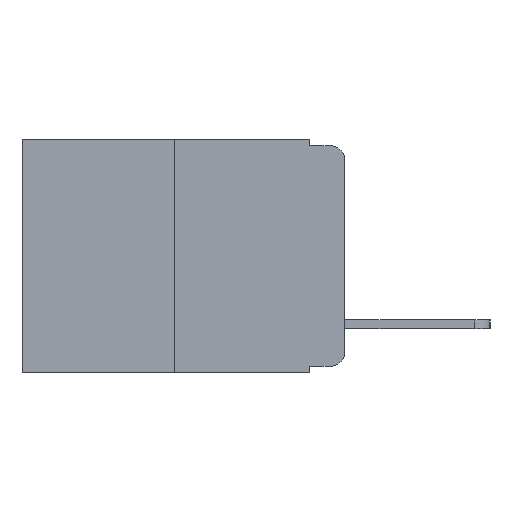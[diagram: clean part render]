
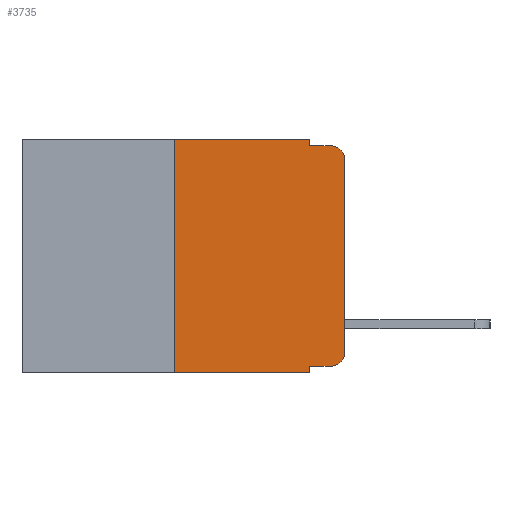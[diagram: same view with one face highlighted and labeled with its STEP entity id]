
A CAD part, left-side view. The second image highlights one B-rep face of the part: STEP entity #3735.
In plain terms, the highlighted planar face has unit normal (-1, 0, 0).
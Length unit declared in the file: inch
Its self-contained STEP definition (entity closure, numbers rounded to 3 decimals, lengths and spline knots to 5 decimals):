
#361 = FACE_OUTER_BOUND ( 'NONE', #10291, .T. ) ;
#640 = LINE ( 'NONE', #11534, #10265 ) ;
#1493 = ORIENTED_EDGE ( 'NONE', *, *, #13781, .T. ) ;
#2721 = EDGE_CURVE ( 'NONE', #24063, #6639, #3100, .T. ) ;
#3065 = ORIENTED_EDGE ( 'NONE', *, *, #8632, .F. ) ;
#3100 = CIRCLE ( 'NONE', #19921, 0.02 ) ;
#3226 = LINE ( 'NONE', #7945, #12706 ) ;
#3735 = ADVANCED_FACE ( 'NONE', ( #361 ), #19083, .F. ) ;
#3847 = DIRECTION ( 'NONE',  ( 0., 0., -1. ) ) ;
#4393 = DIRECTION ( 'NONE',  ( 0., -1., 0. ) ) ;
#4497 = CARTESIAN_POINT ( 'NONE',  ( 0., 0.051, 0. ) ) ;
#4595 = DIRECTION ( 'NONE',  ( 0., -1., 0. ) ) ;
#5886 = CARTESIAN_POINT ( 'NONE',  ( 0., 0.051, -0.333 ) ) ;
#6579 = VECTOR ( 'NONE', #8609, 39.37008 ) ;
#6639 = VERTEX_POINT ( 'NONE', #22176 ) ;
#6747 = CARTESIAN_POINT ( 'NONE',  ( 0., 0.473, 0. ) ) ;
#7032 = ORIENTED_EDGE ( 'NONE', *, *, #11945, .T. ) ;
#7198 = ORIENTED_EDGE ( 'NONE', *, *, #11677, .T. ) ;
#7813 = DIRECTION ( 'NONE',  ( 0., 0., 1. ) ) ;
#7945 = CARTESIAN_POINT ( 'NONE',  ( 0., 0.051, 0. ) ) ;
#8054 = DIRECTION ( 'NONE',  ( -1., 0., 0. ) ) ;
#8243 = CARTESIAN_POINT ( 'NONE',  ( 0., 0.473, -0.343 ) ) ;
#8609 = DIRECTION ( 'NONE',  ( 0., 0., 1. ) ) ;
#8632 = EDGE_CURVE ( 'NONE', #16988, #13642, #3226, .T. ) ;
#8812 = CIRCLE ( 'NONE', #11012, 0.02 ) ;
#9654 = VERTEX_POINT ( 'NONE', #13402 ) ;
#9735 = LINE ( 'NONE', #6747, #19021 ) ;
#10265 = VECTOR ( 'NONE', #7813, 39.37008 ) ;
#10291 = EDGE_LOOP ( 'NONE', ( #7032, #1493, #15149, #3065, #13719, #16018, #7198, #15300, #17335, #17017 ) ) ;
#10590 = DIRECTION ( 'NONE',  ( 0., -1., 0. ) ) ;
#10870 = EDGE_CURVE ( 'NONE', #9654, #13941, #19320, .T. ) ;
#11012 = AXIS2_PLACEMENT_3D ( 'NONE', #19149, #8054, #21057 ) ;
#11194 = CARTESIAN_POINT ( 'NONE',  ( 0., 0.02, -0.333 ) ) ;
#11440 = VERTEX_POINT ( 'NONE', #16772 ) ;
#11534 = CARTESIAN_POINT ( 'NONE',  ( 0., 0., 0. ) ) ;
#11677 = EDGE_CURVE ( 'NONE', #13346, #13941, #21666, .T. ) ;
#11911 = VECTOR ( 'NONE', #4393, 39.37008 ) ;
#11945 = EDGE_CURVE ( 'NONE', #6639, #23827, #640, .T. ) ;
#12223 = CARTESIAN_POINT ( 'NONE',  ( 0., 0.051, -0.343 ) ) ;
#12706 = VECTOR ( 'NONE', #19039, 39.37008 ) ;
#13047 = CARTESIAN_POINT ( 'NONE',  ( 0., 0.051, -0.01 ) ) ;
#13346 = VERTEX_POINT ( 'NONE', #21586 ) ;
#13402 = CARTESIAN_POINT ( 'NONE',  ( 0., 0.051, -0.333 ) ) ;
#13642 = VERTEX_POINT ( 'NONE', #13047 ) ;
#13719 = ORIENTED_EDGE ( 'NONE', *, *, #18141, .F. ) ;
#13779 = VECTOR ( 'NONE', #3847, 39.37008 ) ;
#13781 = EDGE_CURVE ( 'NONE', #23827, #11440, #8812, .T. ) ;
#13941 = VERTEX_POINT ( 'NONE', #12223 ) ;
#14936 = CARTESIAN_POINT ( 'NONE',  ( 0., 0.473, 0. ) ) ;
#15043 = EDGE_CURVE ( 'NONE', #9654, #24063, #21846, .T. ) ;
#15149 = ORIENTED_EDGE ( 'NONE', *, *, #20105, .F. ) ;
#15300 = ORIENTED_EDGE ( 'NONE', *, *, #10870, .F. ) ;
#15318 = DIRECTION ( 'NONE',  ( 0., 0., -1. ) ) ;
#15418 = DIRECTION ( 'NONE',  ( -1., 0., 0. ) ) ;
#15557 = DIRECTION ( 'NONE',  ( 0., -1., 0. ) ) ;
#15718 = VERTEX_POINT ( 'NONE', #19155 ) ;
#15730 = CARTESIAN_POINT ( 'NONE',  ( 0., 0.02, -0.313 ) ) ;
#16018 = ORIENTED_EDGE ( 'NONE', *, *, #24380, .F. ) ;
#16613 = VECTOR ( 'NONE', #15557, 39.37008 ) ;
#16772 = CARTESIAN_POINT ( 'NONE',  ( 0., 0.02, -0.01 ) ) ;
#16885 = CARTESIAN_POINT ( 'NONE',  ( 0., 0.051, 0. ) ) ;
#16988 = VERTEX_POINT ( 'NONE', #4497 ) ;
#17017 = ORIENTED_EDGE ( 'NONE', *, *, #2721, .T. ) ;
#17335 = ORIENTED_EDGE ( 'NONE', *, *, #15043, .T. ) ;
#17725 = CARTESIAN_POINT ( 'NONE',  ( 0., 0.051, -0.01 ) ) ;
#17857 = CARTESIAN_POINT ( 'NONE',  ( 0., 0., -0.03 ) ) ;
#18141 = EDGE_CURVE ( 'NONE', #15718, #16988, #9735, .T. ) ;
#18396 = VECTOR ( 'NONE', #4595, 39.37008 ) ;
#18496 = LINE ( 'NONE', #19711, #6579 ) ;
#19021 = VECTOR ( 'NONE', #10590, 39.37008 ) ;
#19039 = DIRECTION ( 'NONE',  ( 0., 0., -1. ) ) ;
#19083 = PLANE ( 'NONE',  #19308 ) ;
#19149 = CARTESIAN_POINT ( 'NONE',  ( 0., 0.02, -0.03 ) ) ;
#19155 = CARTESIAN_POINT ( 'NONE',  ( 0., 0.25, 0. ) ) ;
#19308 = AXIS2_PLACEMENT_3D ( 'NONE', #14936, #22792, #22763 ) ;
#19320 = LINE ( 'NONE', #16885, #13779 ) ;
#19711 = CARTESIAN_POINT ( 'NONE',  ( 0., 0.25, 0. ) ) ;
#19921 = AXIS2_PLACEMENT_3D ( 'NONE', #15730, #15418, #15318 ) ;
#20105 = EDGE_CURVE ( 'NONE', #13642, #11440, #20772, .T. ) ;
#20772 = LINE ( 'NONE', #17725, #18396 ) ;
#21057 = DIRECTION ( 'NONE',  ( 0., 0., -1. ) ) ;
#21586 = CARTESIAN_POINT ( 'NONE',  ( 0., 0.25, -0.343 ) ) ;
#21666 = LINE ( 'NONE', #8243, #16613 ) ;
#21846 = LINE ( 'NONE', #5886, #11911 ) ;
#22176 = CARTESIAN_POINT ( 'NONE',  ( 0., 0., -0.313 ) ) ;
#22763 = DIRECTION ( 'NONE',  ( 0., 0., -1. ) ) ;
#22792 = DIRECTION ( 'NONE',  ( 1., 0., 0. ) ) ;
#23827 = VERTEX_POINT ( 'NONE', #17857 ) ;
#24063 = VERTEX_POINT ( 'NONE', #11194 ) ;
#24380 = EDGE_CURVE ( 'NONE', #13346, #15718, #18496, .T. ) ;
